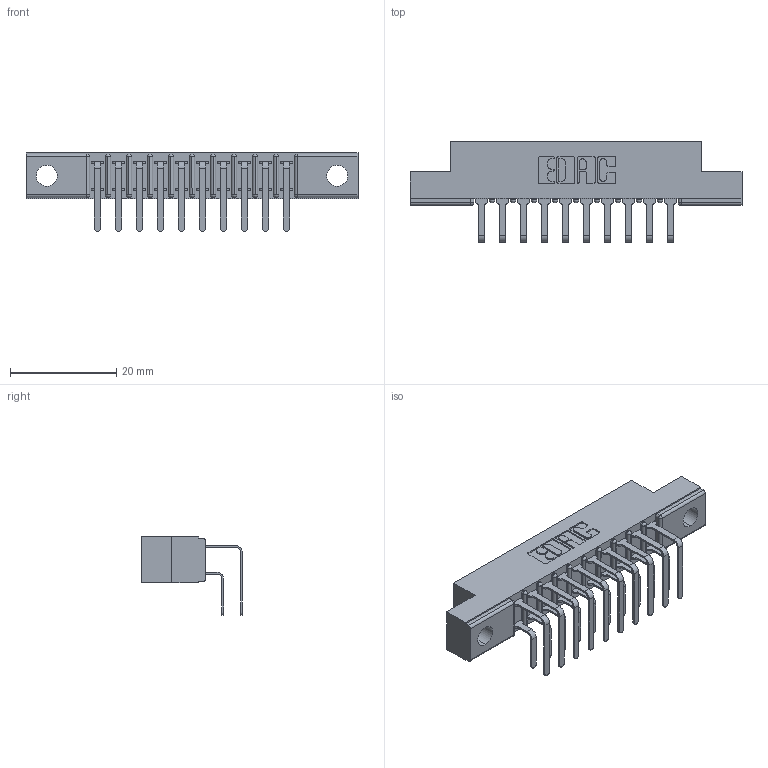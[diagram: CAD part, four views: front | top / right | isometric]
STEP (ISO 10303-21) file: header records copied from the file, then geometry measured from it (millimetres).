
FILE_DESCRIPTION (( 'STEP AP203' ), '1' );
FILE_NAME ('307-010-458-104.STEP', '2020-09-25T07:32:02', ( '' ), ( '' ), 'SwSTEP 2.0', 'SolidWorks 2020', '' );
FILE_SCHEMA (( 'CONFIG_CONTROL_DESIGN' ));
Length unit declared in the file: inch
Products named in the file (4): 307-010-458-104; 307 Part_.156 Dia Mounting Holes; 307-290-001_558 559 - 1 (Single); 307-290-001_558 - 2 (Single)
Assembly tree (21 placements, depth 2):
  307-010-458-104
    307 Part_.156 Dia Mounting Holes
    307-290-001_558 559 - 1 (Single)  x10
    307-290-001_558 - 2 (Single)  x10
Bounding box: 62.64 x 18.96 x 14.81 mm (x, y, z)
Volume: 4081.2 mm3; surface area: 6970.1 mm2
Topology: 21 solids, 21 shells, 1143 faces, 3199 edges, 2074 vertices
Faces by surface type: plane 744, cylinder 377, sphere 22
Entity records: 14703 total; most frequent: CARTESIAN_POINT 2422, ORIENTED_EDGE 2394, DIRECTION 2377, EDGE_CURVE 1197, VECTOR 911, LINE 911, VERTEX_POINT 778, AXIS2_PLACEMENT_3D 733
